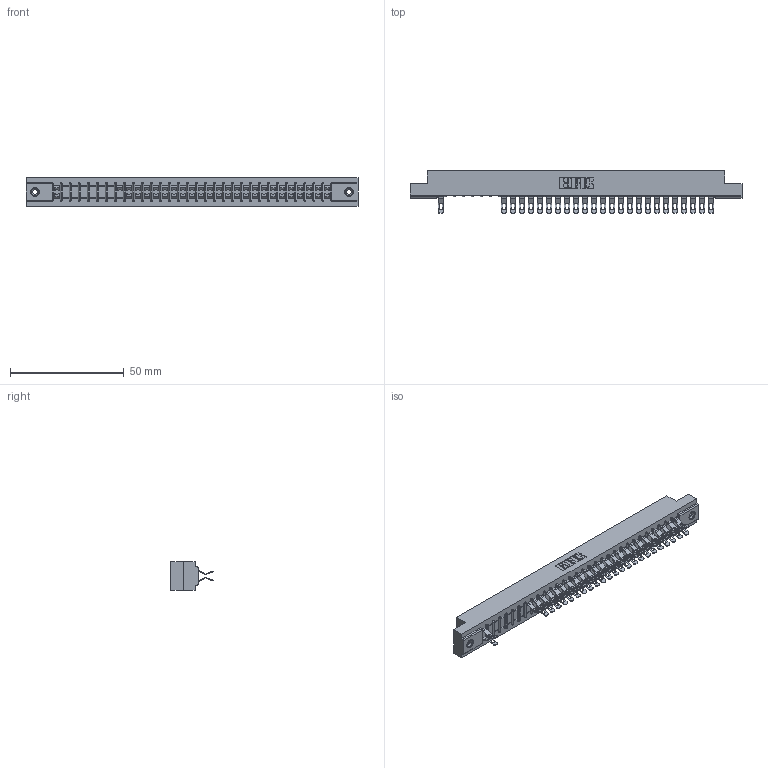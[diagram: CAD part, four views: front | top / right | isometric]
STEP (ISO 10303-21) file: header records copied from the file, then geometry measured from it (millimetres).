
FILE_DESCRIPTION (( 'STEP AP203' ), '1' );
FILE_NAME ('307-062-555-208.STEP', '2018-08-06T09:27:49', ( '' ), ( '' ), 'SwSTEP 2.0', 'SolidWorks 2016', '' );
FILE_SCHEMA (( 'CONFIG_CONTROL_DESIGN' ));
Length unit declared in the file: inch
Products named in the file (4): 307 Part_.156 Dia Mounting Holes; 307-290-001_555; 345-250-001_345-250-003-102; 307-062-555-208
Assembly tree (52 placements, depth 2):
  307-062-555-208
    307 Part_.156 Dia Mounting Holes
    307-290-001_555  x49
    345-250-001_345-250-003-102  x2
Bounding box: 145.85 x 18.75 x 12.7 mm (x, y, z)
Volume: 15402.3 mm3; surface area: 18349.2 mm2
Topology: 52 solids, 52 shells, 3329 faces, 9744 edges, 6336 vertices
Faces by surface type: plane 1846, cylinder 1403, sphere 64, cone 12, torus 4
Entity records: 30230 total; most frequent: CARTESIAN_POINT 4993, ORIENTED_EDGE 4956, DIRECTION 4898, EDGE_CURVE 2478, VECTOR 1884, LINE 1884, VERTEX_POINT 1602, AXIS2_PLACEMENT_3D 1507
